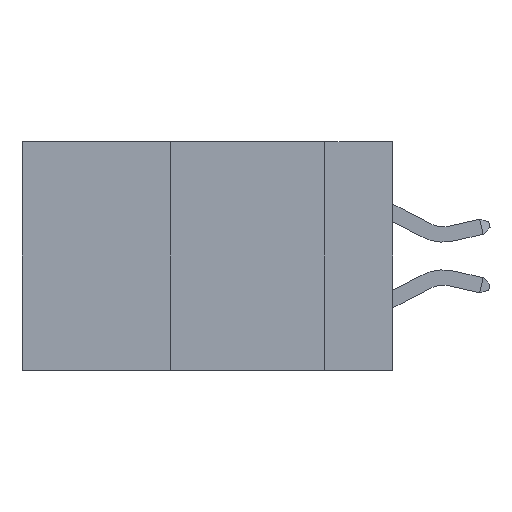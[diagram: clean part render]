
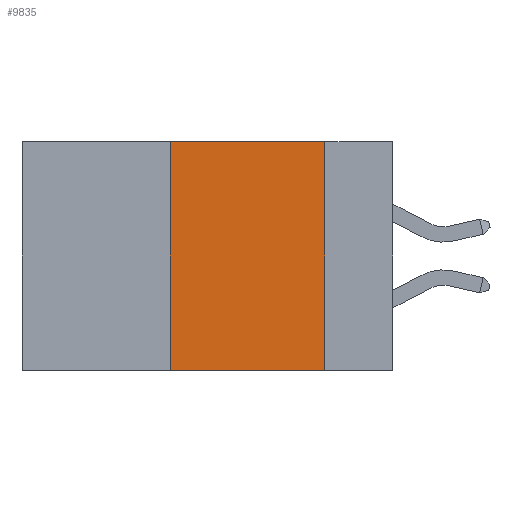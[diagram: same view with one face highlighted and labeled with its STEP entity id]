
A CAD part, left-side view. The second image highlights one B-rep face of the part: STEP entity #9835.
In plain terms, the highlighted planar face has unit normal (-1, 0, 0).
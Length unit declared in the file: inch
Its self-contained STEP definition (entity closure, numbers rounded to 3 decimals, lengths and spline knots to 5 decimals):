
#204 = CARTESIAN_POINT ( 'NONE',  ( 0., 0.11, -0.37 ) ) ;
#791 = LINE ( 'NONE', #30367, #9485 ) ;
#2385 = EDGE_LOOP ( 'NONE', ( #32963, #37905, #22433, #24450 ) ) ;
#2688 = EDGE_CURVE ( 'NONE', #16175, #33083, #27857, .T. ) ;
#4703 = CARTESIAN_POINT ( 'NONE',  ( 0., 0.6, 0. ) ) ;
#6009 = LINE ( 'NONE', #6849, #30799 ) ;
#6849 = CARTESIAN_POINT ( 'NONE',  ( 0., 0.36, 0. ) ) ;
#7257 = CARTESIAN_POINT ( 'NONE',  ( 0., 0.11, 0. ) ) ;
#7773 = DIRECTION ( 'NONE',  ( 0., -1., 0. ) ) ;
#9485 = VECTOR ( 'NONE', #7773, 39.37008 ) ;
#9530 = CARTESIAN_POINT ( 'NONE',  ( 0., 0.36, -0.37 ) ) ;
#9835 = ADVANCED_FACE ( 'NONE', ( #39658 ), #14553, .F. ) ;
#10556 = EDGE_CURVE ( 'NONE', #23237, #16175, #31674, .T. ) ;
#13723 = CARTESIAN_POINT ( 'NONE',  ( 0., 0.36, 0. ) ) ;
#14553 = PLANE ( 'NONE',  #35487 ) ;
#15597 = EDGE_CURVE ( 'NONE', #19369, #23237, #6009, .T. ) ;
#16175 = VERTEX_POINT ( 'NONE', #31804 ) ;
#17783 = DIRECTION ( 'NONE',  ( 1., 0., 0. ) ) ;
#19369 = VERTEX_POINT ( 'NONE', #9530 ) ;
#22433 = ORIENTED_EDGE ( 'NONE', *, *, #15597, .F. ) ;
#23237 = VERTEX_POINT ( 'NONE', #13723 ) ;
#24450 = ORIENTED_EDGE ( 'NONE', *, *, #27410, .T. ) ;
#24913 = DIRECTION ( 'NONE',  ( 0., -1., 0. ) ) ;
#26630 = DIRECTION ( 'NONE',  ( 0., 0., -1. ) ) ;
#27410 = EDGE_CURVE ( 'NONE', #19369, #33083, #791, .T. ) ;
#27857 = LINE ( 'NONE', #7257, #28860 ) ;
#28860 = VECTOR ( 'NONE', #26630, 39.37008 ) ;
#30367 = CARTESIAN_POINT ( 'NONE',  ( 0., 0.6, -0.37 ) ) ;
#30799 = VECTOR ( 'NONE', #32706, 39.37008 ) ;
#31228 = CARTESIAN_POINT ( 'NONE',  ( 0., 0.6, 0. ) ) ;
#31674 = LINE ( 'NONE', #31228, #38116 ) ;
#31804 = CARTESIAN_POINT ( 'NONE',  ( 0., 0.11, 0. ) ) ;
#32706 = DIRECTION ( 'NONE',  ( 0., 0., 1. ) ) ;
#32963 = ORIENTED_EDGE ( 'NONE', *, *, #2688, .F. ) ;
#33083 = VERTEX_POINT ( 'NONE', #204 ) ;
#35487 = AXIS2_PLACEMENT_3D ( 'NONE', #4703, #17783, #40125 ) ;
#37905 = ORIENTED_EDGE ( 'NONE', *, *, #10556, .F. ) ;
#38116 = VECTOR ( 'NONE', #24913, 39.37008 ) ;
#39658 = FACE_OUTER_BOUND ( 'NONE', #2385, .T. ) ;
#40125 = DIRECTION ( 'NONE',  ( 0., 0., -1. ) ) ;
